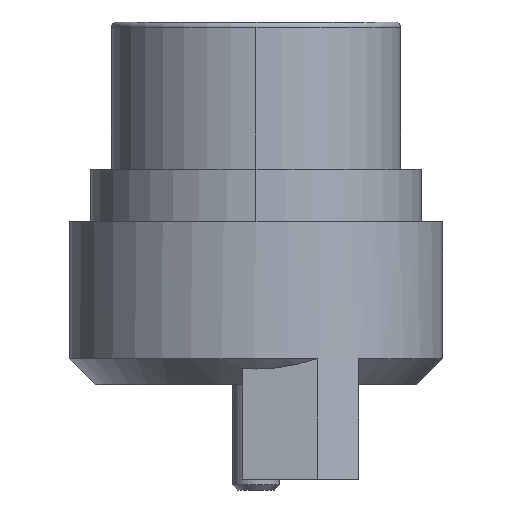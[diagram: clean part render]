
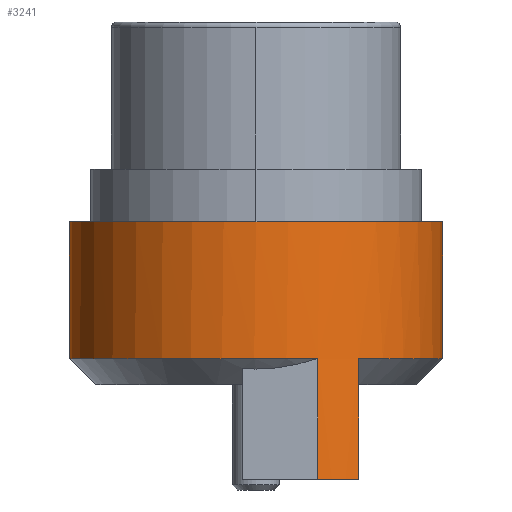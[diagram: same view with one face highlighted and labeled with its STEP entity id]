
A CAD part, left-side view. The second image highlights one B-rep face of the part: STEP entity #3241.
In plain terms, the highlighted cylindrical face has radius 3.55 mm (diameter 7.1 mm), a partial arc.
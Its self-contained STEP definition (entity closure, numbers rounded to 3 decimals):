
#3 = CARTESIAN_POINT ( 'NONE',  ( -5.8, 36.45, -3.8 ) ) ;
#86 = VERTEX_POINT ( 'NONE', #3393 ) ;
#171 = ORIENTED_EDGE ( 'NONE', *, *, #4500, .F. ) ;
#184 = DIRECTION ( 'NONE',  ( -0.836, -0.549, 0. ) ) ;
#204 = CARTESIAN_POINT ( 'NONE',  ( -5.8, 43.55, -3.8 ) ) ;
#211 = CYLINDRICAL_SURFACE ( 'NONE', #3274, 3.55 ) ;
#212 = AXIS2_PLACEMENT_3D ( 'NONE', #2456, #4293, #184 ) ;
#252 = CARTESIAN_POINT ( 'NONE',  ( -5.8, 40., -8.7 ) ) ;
#357 = VERTEX_POINT ( 'NONE', #3 ) ;
#578 = CIRCLE ( 'NONE', #3938, 3.55 ) ;
#589 = DIRECTION ( 'NONE',  ( 0., 0., 1. ) ) ;
#747 = CARTESIAN_POINT ( 'NONE',  ( -5.8, 36.45, -3.8 ) ) ;
#770 = CARTESIAN_POINT ( 'NONE',  ( -9.15, 38.825, -8.7 ) ) ;
#883 = EDGE_CURVE ( 'NONE', #949, #357, #2027, .T. ) ;
#889 = ORIENTED_EDGE ( 'NONE', *, *, #4334, .F. ) ;
#949 = VERTEX_POINT ( 'NONE', #204 ) ;
#952 = VERTEX_POINT ( 'NONE', #2020 ) ;
#1020 = LINE ( 'NONE', #2859, #1592 ) ;
#1077 = LINE ( 'NONE', #2913, #3207 ) ;
#1301 = VECTOR ( 'NONE', #2600, 1000. ) ;
#1360 = ORIENTED_EDGE ( 'NONE', *, *, #883, .F. ) ;
#1522 = VERTEX_POINT ( 'NONE', #4424 ) ;
#1544 = DIRECTION ( 'NONE',  ( 0., 0., 1. ) ) ;
#1592 = VECTOR ( 'NONE', #4696, 1000. ) ;
#1865 = AXIS2_PLACEMENT_3D ( 'NONE', #5674, #1544, #3383 ) ;
#2020 = CARTESIAN_POINT ( 'NONE',  ( -5.8, 43.55, -6.4 ) ) ;
#2027 = CIRCLE ( 'NONE', #2802, 3.55 ) ;
#2030 = CARTESIAN_POINT ( 'NONE',  ( -5.8, 40., -8.798 ) ) ;
#2069 = DIRECTION ( 'NONE',  ( 0., 0., -1. ) ) ;
#2251 = EDGE_CURVE ( 'NONE', #952, #949, #1077, .T. ) ;
#2413 = DIRECTION ( 'NONE',  ( 0., 1., 0. ) ) ;
#2456 = CARTESIAN_POINT ( 'NONE',  ( -5.8, 40., -6.4 ) ) ;
#2577 = DIRECTION ( 'NONE',  ( 0., 0., -1. ) ) ;
#2600 = DIRECTION ( 'NONE',  ( 0., 0., 1. ) ) ;
#2638 = EDGE_CURVE ( 'NONE', #1522, #86, #578, .T. ) ;
#2749 = ORIENTED_EDGE ( 'NONE', *, *, #3782, .F. ) ;
#2798 = CIRCLE ( 'NONE', #212, 3.55 ) ;
#2802 = AXIS2_PLACEMENT_3D ( 'NONE', #4710, #589, #2413 ) ;
#2806 = EDGE_LOOP ( 'NONE', ( #1360, #5780, #5909, #2749, #5673, #889, #4642, #171 ) ) ;
#2859 = CARTESIAN_POINT ( 'NONE',  ( -8.766, 38.05, -6.4 ) ) ;
#2913 = CARTESIAN_POINT ( 'NONE',  ( -5.8, 43.55, -6.4 ) ) ;
#3193 = EDGE_CURVE ( 'NONE', #5868, #3306, #2798, .T. ) ;
#3207 = VECTOR ( 'NONE', #4747, 1000. ) ;
#3241 = ADVANCED_FACE ( 'NONE', ( #4319 ), #211, .T. ) ;
#3274 = AXIS2_PLACEMENT_3D ( 'NONE', #2030, #3874, #5705 ) ;
#3306 = VERTEX_POINT ( 'NONE', #3961 ) ;
#3383 = DIRECTION ( 'NONE',  ( 0., 1., 0. ) ) ;
#3393 = CARTESIAN_POINT ( 'NONE',  ( -9.15, 38.825, -8.7 ) ) ;
#3671 = EDGE_CURVE ( 'NONE', #952, #4825, #4471, .T. ) ;
#3782 = EDGE_CURVE ( 'NONE', #86, #4825, #4895, .T. ) ;
#3874 = DIRECTION ( 'NONE',  ( 0., 0., 1. ) ) ;
#3917 = DIRECTION ( 'NONE',  ( -0.836, -0.549, 0. ) ) ;
#3938 = AXIS2_PLACEMENT_3D ( 'NONE', #252, #2069, #3917 ) ;
#3961 = CARTESIAN_POINT ( 'NONE',  ( -5.8, 36.45, -6.4 ) ) ;
#4151 = CARTESIAN_POINT ( 'NONE',  ( -9.15, 38.825, -6.4 ) ) ;
#4293 = DIRECTION ( 'NONE',  ( 0., 0., 1. ) ) ;
#4319 = FACE_OUTER_BOUND ( 'NONE', #2806, .T. ) ;
#4334 = EDGE_CURVE ( 'NONE', #5868, #1522, #1020, .T. ) ;
#4424 = CARTESIAN_POINT ( 'NONE',  ( -8.766, 38.05, -8.7 ) ) ;
#4471 = CIRCLE ( 'NONE', #1865, 3.55 ) ;
#4500 = EDGE_CURVE ( 'NONE', #357, #3306, #4872, .T. ) ;
#4586 = VECTOR ( 'NONE', #2577, 1000. ) ;
#4642 = ORIENTED_EDGE ( 'NONE', *, *, #3193, .T. ) ;
#4696 = DIRECTION ( 'NONE',  ( 0., 0., -1. ) ) ;
#4710 = CARTESIAN_POINT ( 'NONE',  ( -5.8, 40., -3.8 ) ) ;
#4747 = DIRECTION ( 'NONE',  ( 0., 0., 1. ) ) ;
#4825 = VERTEX_POINT ( 'NONE', #4151 ) ;
#4872 = LINE ( 'NONE', #747, #4586 ) ;
#4895 = LINE ( 'NONE', #770, #1301 ) ;
#5224 = CARTESIAN_POINT ( 'NONE',  ( -8.766, 38.05, -6.4 ) ) ;
#5673 = ORIENTED_EDGE ( 'NONE', *, *, #2638, .F. ) ;
#5674 = CARTESIAN_POINT ( 'NONE',  ( -5.8, 40., -6.4 ) ) ;
#5705 = DIRECTION ( 'NONE',  ( 1., 0., 0. ) ) ;
#5780 = ORIENTED_EDGE ( 'NONE', *, *, #2251, .F. ) ;
#5868 = VERTEX_POINT ( 'NONE', #5224 ) ;
#5909 = ORIENTED_EDGE ( 'NONE', *, *, #3671, .T. ) ;
